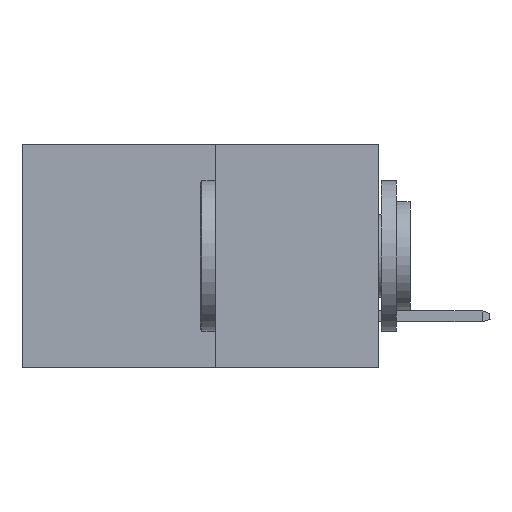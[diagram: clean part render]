
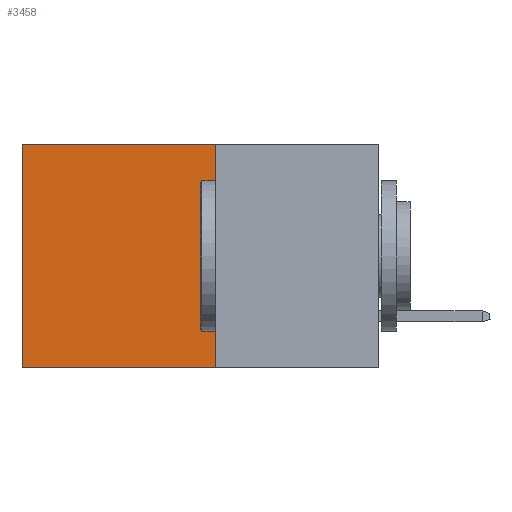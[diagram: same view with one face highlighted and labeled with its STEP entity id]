
A CAD part, left-side view. The second image highlights one B-rep face of the part: STEP entity #3458.
In plain terms, the highlighted planar face has unit normal (-1, 0, 0).
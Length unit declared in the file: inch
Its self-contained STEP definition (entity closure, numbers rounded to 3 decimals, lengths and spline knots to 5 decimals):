
#3099 = CARTESIAN_POINT ( 'NONE',  ( 0.277, 0.59, -0.37 ) ) ;
#3458 = ADVANCED_FACE ( 'NONE', ( #3902 ), #31139, .F. ) ;
#3902 = FACE_OUTER_BOUND ( 'NONE', #24656, .T. ) ;
#4010 = VECTOR ( 'NONE', #16071, 39.37008 ) ;
#4292 = VERTEX_POINT ( 'NONE', #9061 ) ;
#4845 = LINE ( 'NONE', #3099, #4010 ) ;
#5385 = DIRECTION ( 'NONE',  ( 0., 1., 0. ) ) ;
#5843 = CARTESIAN_POINT ( 'NONE',  ( 0.277, 0.27, 0. ) ) ;
#8089 = EDGE_CURVE ( 'NONE', #25460, #4292, #26033, .T. ) ;
#8138 = VECTOR ( 'NONE', #5385, 39.37008 ) ;
#8420 = CARTESIAN_POINT ( 'NONE',  ( 0.277, 0.27, 0. ) ) ;
#8772 = EDGE_CURVE ( 'NONE', #22891, #19909, #4845, .T. ) ;
#9061 = CARTESIAN_POINT ( 'NONE',  ( 0.277, 0.27, -0.37 ) ) ;
#10480 = AXIS2_PLACEMENT_3D ( 'NONE', #31183, #31104, #31101 ) ;
#10952 = CARTESIAN_POINT ( 'NONE',  ( 0.277, 0.27, -0.37 ) ) ;
#12216 = EDGE_CURVE ( 'NONE', #4292, #19909, #14991, .T. ) ;
#13821 = ORIENTED_EDGE ( 'NONE', *, *, #8772, .T. ) ;
#14991 = LINE ( 'NONE', #15688, #8138 ) ;
#15688 = CARTESIAN_POINT ( 'NONE',  ( 0.277, 0.27, -0.37 ) ) ;
#16071 = DIRECTION ( 'NONE',  ( 0., 0., -1. ) ) ;
#16873 = ORIENTED_EDGE ( 'NONE', *, *, #8089, .F. ) ;
#18351 = VECTOR ( 'NONE', #29096, 39.37008 ) ;
#19909 = VERTEX_POINT ( 'NONE', #29082 ) ;
#22891 = VERTEX_POINT ( 'NONE', #26244 ) ;
#23776 = ORIENTED_EDGE ( 'NONE', *, *, #24769, .T. ) ;
#24656 = EDGE_LOOP ( 'NONE', ( #13821, #31685, #16873, #23776 ) ) ;
#24769 = EDGE_CURVE ( 'NONE', #25460, #22891, #25287, .T. ) ;
#25219 = VECTOR ( 'NONE', #31528, 39.37008 ) ;
#25287 = LINE ( 'NONE', #8420, #18351 ) ;
#25460 = VERTEX_POINT ( 'NONE', #5843 ) ;
#26033 = LINE ( 'NONE', #10952, #25219 ) ;
#26244 = CARTESIAN_POINT ( 'NONE',  ( 0.277, 0.59, 0. ) ) ;
#29082 = CARTESIAN_POINT ( 'NONE',  ( 0.277, 0.59, -0.37 ) ) ;
#29096 = DIRECTION ( 'NONE',  ( 0., 1., 0. ) ) ;
#31101 = DIRECTION ( 'NONE',  ( 0., 0., -1. ) ) ;
#31104 = DIRECTION ( 'NONE',  ( 1., 0., 0. ) ) ;
#31139 = PLANE ( 'NONE',  #10480 ) ;
#31183 = CARTESIAN_POINT ( 'NONE',  ( 0.277, 0.27, -0.37 ) ) ;
#31528 = DIRECTION ( 'NONE',  ( 0., 0., -1. ) ) ;
#31685 = ORIENTED_EDGE ( 'NONE', *, *, #12216, .F. ) ;
